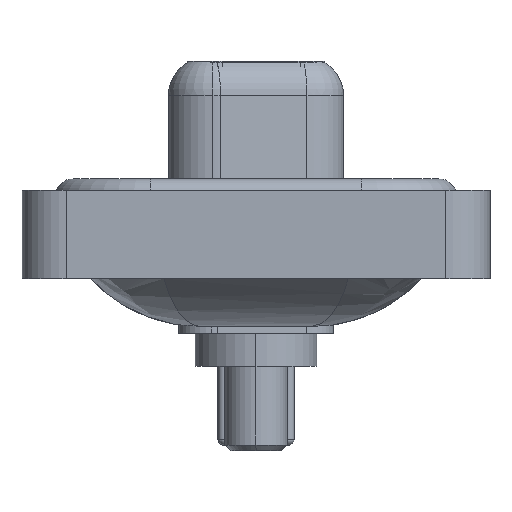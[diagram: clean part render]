
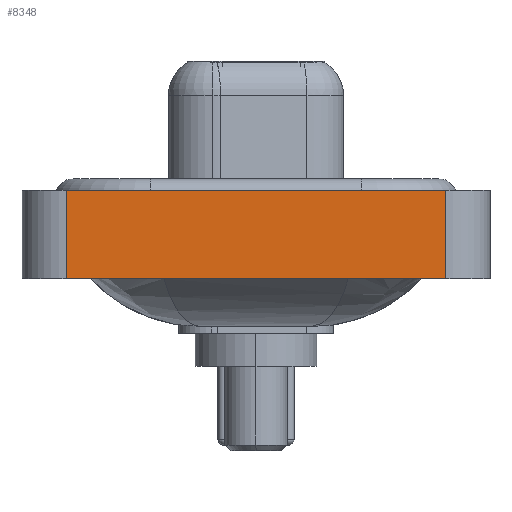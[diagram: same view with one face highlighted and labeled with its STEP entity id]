
A CAD part, left-side view. The second image highlights one B-rep face of the part: STEP entity #8348.
In plain terms, the highlighted planar face has unit normal (-1, 0, 0).
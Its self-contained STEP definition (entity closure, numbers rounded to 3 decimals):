
#928 = VERTEX_POINT ( 'NONE', #14802 ) ;
#1954 = VECTOR ( 'NONE', #13300, 1000. ) ;
#2052 = AXIS2_PLACEMENT_3D ( 'NONE', #10904, #8573, #19745 ) ;
#2280 = LINE ( 'NONE', #7903, #1954 ) ;
#3778 = ORIENTED_EDGE ( 'NONE', *, *, #7550, .T. ) ;
#4706 = CARTESIAN_POINT ( 'NONE',  ( -7.35, -8.55, 0.4 ) ) ;
#5199 = DIRECTION ( 'NONE',  ( 0., -1., 0. ) ) ;
#5263 = FACE_OUTER_BOUND ( 'NONE', #10234, .T. ) ;
#5895 = VERTEX_POINT ( 'NONE', #21042 ) ;
#6057 = VERTEX_POINT ( 'NONE', #23131 ) ;
#6394 = ORIENTED_EDGE ( 'NONE', *, *, #10406, .T. ) ;
#7531 = CARTESIAN_POINT ( 'NONE',  ( -7.35, 8.55, -3.6 ) ) ;
#7550 = EDGE_CURVE ( 'NONE', #928, #5895, #14780, .T. ) ;
#7756 = DIRECTION ( 'NONE',  ( 0., 0., 1. ) ) ;
#7903 = CARTESIAN_POINT ( 'NONE',  ( -7.35, -8.55, -3.6 ) ) ;
#8348 = ADVANCED_FACE ( 'NONE', ( #5263 ), #23581, .T. ) ;
#8369 = VECTOR ( 'NONE', #7756, 1000. ) ;
#8573 = DIRECTION ( 'NONE',  ( -1., 0., 0. ) ) ;
#9099 = VERTEX_POINT ( 'NONE', #4706 ) ;
#9291 = VECTOR ( 'NONE', #11323, 1000. ) ;
#9500 = LINE ( 'NONE', #13290, #9291 ) ;
#10234 = EDGE_LOOP ( 'NONE', ( #6394, #18004, #23882, #3778 ) ) ;
#10406 = EDGE_CURVE ( 'NONE', #5895, #9099, #2280, .T. ) ;
#10904 = CARTESIAN_POINT ( 'NONE',  ( -7.35, -8.55, -3.6 ) ) ;
#11323 = DIRECTION ( 'NONE',  ( 0., -1., 0. ) ) ;
#12313 = EDGE_CURVE ( 'NONE', #928, #6057, #16870, .T. ) ;
#13290 = CARTESIAN_POINT ( 'NONE',  ( -7.35, -8.55, 0.4 ) ) ;
#13300 = DIRECTION ( 'NONE',  ( 0., 0., 1. ) ) ;
#14272 = CARTESIAN_POINT ( 'NONE',  ( -7.35, -8.55, -3.6 ) ) ;
#14780 = LINE ( 'NONE', #14272, #18477 ) ;
#14802 = CARTESIAN_POINT ( 'NONE',  ( -7.35, 8.55, -3.6 ) ) ;
#16870 = LINE ( 'NONE', #7531, #8369 ) ;
#18004 = ORIENTED_EDGE ( 'NONE', *, *, #18802, .F. ) ;
#18477 = VECTOR ( 'NONE', #5199, 1000. ) ;
#18802 = EDGE_CURVE ( 'NONE', #6057, #9099, #9500, .T. ) ;
#19745 = DIRECTION ( 'NONE',  ( 0., 0., 1. ) ) ;
#21042 = CARTESIAN_POINT ( 'NONE',  ( -7.35, -8.55, -3.6 ) ) ;
#23131 = CARTESIAN_POINT ( 'NONE',  ( -7.35, 8.55, 0.4 ) ) ;
#23581 = PLANE ( 'NONE',  #2052 ) ;
#23882 = ORIENTED_EDGE ( 'NONE', *, *, #12313, .F. ) ;
